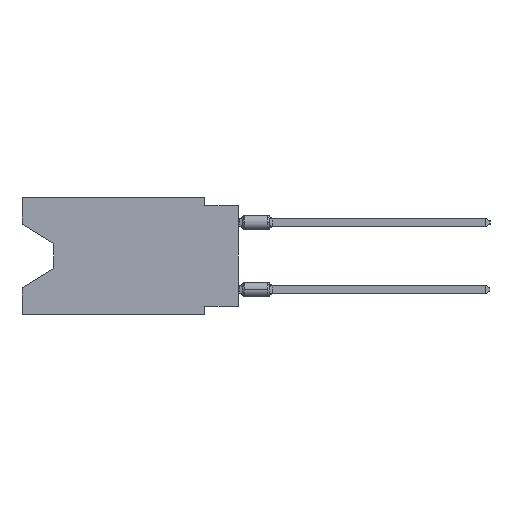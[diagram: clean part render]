
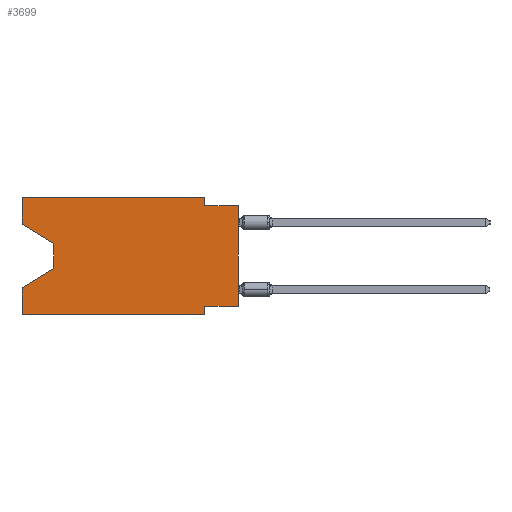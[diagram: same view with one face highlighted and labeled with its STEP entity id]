
A CAD part, left-side view. The second image highlights one B-rep face of the part: STEP entity #3699.
In plain terms, the highlighted planar face has unit normal (-1, 0, 0).
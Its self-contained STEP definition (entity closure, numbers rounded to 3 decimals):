
#442 = DIRECTION ( 'NONE',  ( 0., 0., -1. ) ) ;
#739 = DIRECTION ( 'NONE',  ( 0., 0., 1. ) ) ;
#1406 = CARTESIAN_POINT ( 'NONE',  ( 0., 13.97, -3.505 ) ) ;
#1725 = DIRECTION ( 'NONE',  ( 0., 0., -1. ) ) ;
#2121 = VERTEX_POINT ( 'NONE', #20403 ) ;
#2659 = CARTESIAN_POINT ( 'NONE',  ( 0., 16.383, -2.038 ) ) ;
#3336 = CARTESIAN_POINT ( 'NONE',  ( 0., 13.97, -5.385 ) ) ;
#3699 = ADVANCED_FACE ( 'NONE', ( #36017 ), #30475, .F. ) ;
#5470 = VERTEX_POINT ( 'NONE', #40083 ) ;
#5680 = ORIENTED_EDGE ( 'NONE', *, *, #56204, .F. ) ;
#6278 = EDGE_CURVE ( 'NONE', #7598, #2121, #15436, .T. ) ;
#6288 = CARTESIAN_POINT ( 'NONE',  ( 0., 13.97, -5.385 ) ) ;
#6402 = VERTEX_POINT ( 'NONE', #31097 ) ;
#6772 = DIRECTION ( 'NONE',  ( 0., -1., 0. ) ) ;
#6894 = EDGE_CURVE ( 'NONE', #6402, #2121, #31588, .T. ) ;
#7260 = CARTESIAN_POINT ( 'NONE',  ( 0., 0., -8.255 ) ) ;
#7598 = VERTEX_POINT ( 'NONE', #40590 ) ;
#7794 = DIRECTION ( 'NONE',  ( 0., -1., 0. ) ) ;
#8046 = DIRECTION ( 'NONE',  ( 0., 1., 0. ) ) ;
#8325 = VECTOR ( 'NONE', #8046, 1000. ) ;
#8397 = ORIENTED_EDGE ( 'NONE', *, *, #60848, .F. ) ;
#9062 = LINE ( 'NONE', #28352, #63163 ) ;
#9600 = LINE ( 'NONE', #64462, #53796 ) ;
#9879 = CARTESIAN_POINT ( 'NONE',  ( 0., 16.383, 0. ) ) ;
#10191 = CARTESIAN_POINT ( 'NONE',  ( 0., 2.54, 0. ) ) ;
#10514 = ORIENTED_EDGE ( 'NONE', *, *, #12643, .F. ) ;
#10962 = CARTESIAN_POINT ( 'NONE',  ( 0., 16.383, 0. ) ) ;
#11523 = EDGE_CURVE ( 'NONE', #18382, #25503, #16100, .T. ) ;
#11712 = EDGE_CURVE ( 'NONE', #25503, #59228, #58517, .T. ) ;
#12643 = EDGE_CURVE ( 'NONE', #35303, #5470, #9600, .T. ) ;
#13822 = ORIENTED_EDGE ( 'NONE', *, *, #42168, .T. ) ;
#15403 = EDGE_CURVE ( 'NONE', #52835, #27692, #58434, .T. ) ;
#15436 = LINE ( 'NONE', #35348, #25154 ) ;
#16100 = LINE ( 'NONE', #1406, #25468 ) ;
#18231 = LINE ( 'NONE', #27071, #28002 ) ;
#18382 = VERTEX_POINT ( 'NONE', #40334 ) ;
#18948 = VECTOR ( 'NONE', #6772, 1000. ) ;
#20403 = CARTESIAN_POINT ( 'NONE',  ( 0., 2.54, -8.89 ) ) ;
#20932 = EDGE_CURVE ( 'NONE', #6402, #59228, #39592, .T. ) ;
#23233 = DIRECTION ( 'NONE',  ( 0., 0.855, -0.519 ) ) ;
#25154 = VECTOR ( 'NONE', #60501, 1000. ) ;
#25241 = VECTOR ( 'NONE', #48325, 1000. ) ;
#25468 = VECTOR ( 'NONE', #1725, 1000. ) ;
#25503 = VERTEX_POINT ( 'NONE', #6288 ) ;
#27071 = CARTESIAN_POINT ( 'NONE',  ( 0., 0., -0.635 ) ) ;
#27692 = VERTEX_POINT ( 'NONE', #47908 ) ;
#28002 = VECTOR ( 'NONE', #7794, 1000. ) ;
#28352 = CARTESIAN_POINT ( 'NONE',  ( 0., 16.383, 0. ) ) ;
#30108 = DIRECTION ( 'NONE',  ( 0., 0., -1. ) ) ;
#30475 = PLANE ( 'NONE',  #53290 ) ;
#30529 = CARTESIAN_POINT ( 'NONE',  ( 0., 16.383, -2.038 ) ) ;
#31097 = CARTESIAN_POINT ( 'NONE',  ( 0., 16.383, -8.89 ) ) ;
#31588 = LINE ( 'NONE', #51516, #18948 ) ;
#31778 = VECTOR ( 'NONE', #23233, 1000. ) ;
#31969 = CARTESIAN_POINT ( 'NONE',  ( 0., 2.54, -0.635 ) ) ;
#32871 = CARTESIAN_POINT ( 'NONE',  ( 0., 0., -8.255 ) ) ;
#33918 = ORIENTED_EDGE ( 'NONE', *, *, #15403, .T. ) ;
#34783 = VECTOR ( 'NONE', #40324, 1000. ) ;
#35010 = LINE ( 'NONE', #10191, #57809 ) ;
#35053 = DIRECTION ( 'NONE',  ( 1., 0., 0. ) ) ;
#35303 = VERTEX_POINT ( 'NONE', #10962 ) ;
#35348 = CARTESIAN_POINT ( 'NONE',  ( 0., 2.54, -8.89 ) ) ;
#36017 = FACE_OUTER_BOUND ( 'NONE', #49456, .T. ) ;
#37435 = LINE ( 'NONE', #32871, #8325 ) ;
#37506 = CARTESIAN_POINT ( 'NONE',  ( 0., 16.383, -6.852 ) ) ;
#39548 = ORIENTED_EDGE ( 'NONE', *, *, #11523, .T. ) ;
#39592 = LINE ( 'NONE', #9879, #61572 ) ;
#40083 = CARTESIAN_POINT ( 'NONE',  ( 0., 2.54, 0. ) ) ;
#40324 = DIRECTION ( 'NONE',  ( 0., -0.855, -0.519 ) ) ;
#40334 = CARTESIAN_POINT ( 'NONE',  ( 0., 13.97, -3.505 ) ) ;
#40590 = CARTESIAN_POINT ( 'NONE',  ( 0., 2.54, -8.255 ) ) ;
#40924 = DIRECTION ( 'NONE',  ( 0., -1., 0. ) ) ;
#42168 = EDGE_CURVE ( 'NONE', #47706, #18382, #63554, .T. ) ;
#46556 = ORIENTED_EDGE ( 'NONE', *, *, #20932, .F. ) ;
#46901 = EDGE_CURVE ( 'NONE', #5470, #59015, #35010, .T. ) ;
#47706 = VERTEX_POINT ( 'NONE', #2659 ) ;
#47908 = CARTESIAN_POINT ( 'NONE',  ( 0., 0., -0.635 ) ) ;
#48325 = DIRECTION ( 'NONE',  ( 0., 0., 1. ) ) ;
#48921 = DIRECTION ( 'NONE',  ( 0., 0., 1. ) ) ;
#49010 = ORIENTED_EDGE ( 'NONE', *, *, #6278, .F. ) ;
#49456 = EDGE_LOOP ( 'NONE', ( #13822, #39548, #59583, #46556, #58030, #49010, #8397, #33918, #49869, #61191, #10514, #5680 ) ) ;
#49869 = ORIENTED_EDGE ( 'NONE', *, *, #59117, .F. ) ;
#50085 = CARTESIAN_POINT ( 'NONE',  ( 0., 16.383, 0. ) ) ;
#51516 = CARTESIAN_POINT ( 'NONE',  ( 0., 16.383, -8.89 ) ) ;
#52835 = VERTEX_POINT ( 'NONE', #7260 ) ;
#53290 = AXIS2_PLACEMENT_3D ( 'NONE', #50085, #35053, #442 ) ;
#53796 = VECTOR ( 'NONE', #40924, 1000. ) ;
#56204 = EDGE_CURVE ( 'NONE', #47706, #35303, #9062, .T. ) ;
#57809 = VECTOR ( 'NONE', #30108, 1000. ) ;
#58030 = ORIENTED_EDGE ( 'NONE', *, *, #6894, .T. ) ;
#58434 = LINE ( 'NONE', #58752, #25241 ) ;
#58517 = LINE ( 'NONE', #3336, #31778 ) ;
#58752 = CARTESIAN_POINT ( 'NONE',  ( 0., 0., 0. ) ) ;
#59015 = VERTEX_POINT ( 'NONE', #31969 ) ;
#59117 = EDGE_CURVE ( 'NONE', #59015, #27692, #18231, .T. ) ;
#59228 = VERTEX_POINT ( 'NONE', #37506 ) ;
#59583 = ORIENTED_EDGE ( 'NONE', *, *, #11712, .T. ) ;
#60501 = DIRECTION ( 'NONE',  ( 0., 0., -1. ) ) ;
#60848 = EDGE_CURVE ( 'NONE', #52835, #7598, #37435, .T. ) ;
#61191 = ORIENTED_EDGE ( 'NONE', *, *, #46901, .F. ) ;
#61572 = VECTOR ( 'NONE', #739, 1000. ) ;
#63163 = VECTOR ( 'NONE', #48921, 1000. ) ;
#63554 = LINE ( 'NONE', #30529, #34783 ) ;
#64462 = CARTESIAN_POINT ( 'NONE',  ( 0., 16.383, 0. ) ) ;
